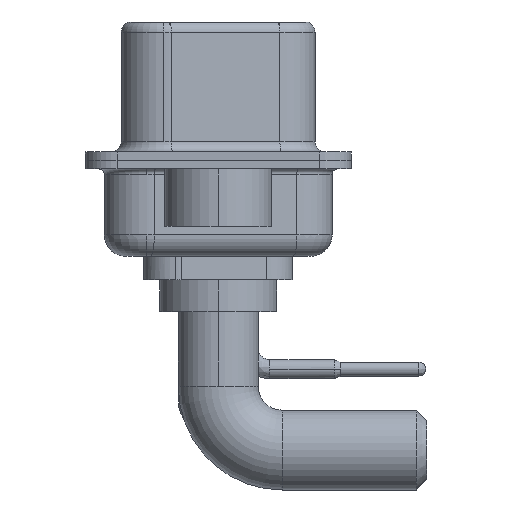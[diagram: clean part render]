
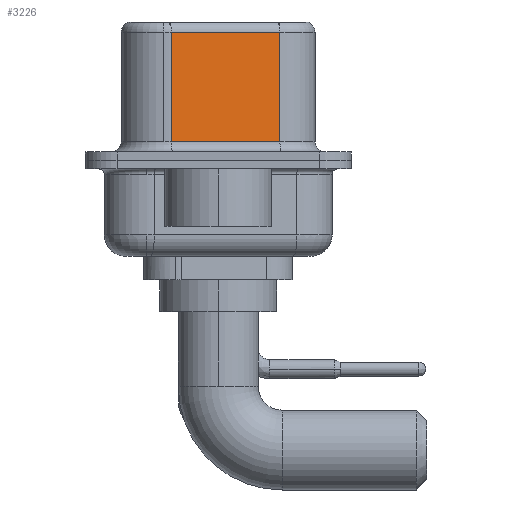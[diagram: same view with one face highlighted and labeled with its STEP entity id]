
A CAD part, left-side view. The second image highlights one B-rep face of the part: STEP entity #3226.
In plain terms, the highlighted planar face has unit normal (-0.985, -0.174, 0).
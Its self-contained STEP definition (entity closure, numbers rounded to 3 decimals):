
#95 = CARTESIAN_POINT ( 'NONE',  ( 4.58, -2.897, 0.9 ) ) ;
#141 = DIRECTION ( 'NONE',  ( 0.985, 0.174, 0. ) ) ;
#1295 = VECTOR ( 'NONE', #1507, 1000. ) ;
#1507 = DIRECTION ( 'NONE',  ( 0., 0., -1. ) ) ;
#2976 = VECTOR ( 'NONE', #14151, 1000. ) ;
#3121 = CARTESIAN_POINT ( 'NONE',  ( 4.58, -2.897, 0.9 ) ) ;
#3226 = ADVANCED_FACE ( 'NONE', ( #17251 ), #7954, .F. ) ;
#4394 = ORIENTED_EDGE ( 'NONE', *, *, #11855, .F. ) ;
#4892 = EDGE_CURVE ( 'NONE', #20461, #14411, #10576, .T. ) ;
#5912 = EDGE_CURVE ( 'NONE', #17487, #20461, #13178, .T. ) ;
#6151 = CARTESIAN_POINT ( 'NONE',  ( 4.58, -2.897, 6.02 ) ) ;
#7954 = PLANE ( 'NONE',  #9165 ) ;
#8474 = LINE ( 'NONE', #3121, #2976 ) ;
#9165 = AXIS2_PLACEMENT_3D ( 'NONE', #10063, #141, #23328 ) ;
#9726 = CARTESIAN_POINT ( 'NONE',  ( 3.68, 2.203, 0.9 ) ) ;
#10063 = CARTESIAN_POINT ( 'NONE',  ( 4.58, -2.897, 6.52 ) ) ;
#10576 = LINE ( 'NONE', #18384, #1295 ) ;
#11517 = CARTESIAN_POINT ( 'NONE',  ( 3.68, 2.203, 6.02 ) ) ;
#11855 = EDGE_CURVE ( 'NONE', #17487, #20853, #12736, .T. ) ;
#12736 = LINE ( 'NONE', #20327, #17567 ) ;
#12982 = DIRECTION ( 'NONE',  ( 0., 0., -1. ) ) ;
#13178 = LINE ( 'NONE', #6151, #18005 ) ;
#14151 = DIRECTION ( 'NONE',  ( 0.174, -0.985, 0. ) ) ;
#14411 = VERTEX_POINT ( 'NONE', #9726 ) ;
#15097 = ORIENTED_EDGE ( 'NONE', *, *, #4892, .T. ) ;
#15219 = EDGE_CURVE ( 'NONE', #14411, #20853, #8474, .T. ) ;
#15337 = ORIENTED_EDGE ( 'NONE', *, *, #5912, .T. ) ;
#17251 = FACE_OUTER_BOUND ( 'NONE', #22195, .T. ) ;
#17487 = VERTEX_POINT ( 'NONE', #18655 ) ;
#17567 = VECTOR ( 'NONE', #12982, 1000. ) ;
#18005 = VECTOR ( 'NONE', #20785, 1000. ) ;
#18384 = CARTESIAN_POINT ( 'NONE',  ( 3.68, 2.203, 6.52 ) ) ;
#18655 = CARTESIAN_POINT ( 'NONE',  ( 4.58, -2.897, 6.02 ) ) ;
#20327 = CARTESIAN_POINT ( 'NONE',  ( 4.58, -2.897, 6.52 ) ) ;
#20384 = ORIENTED_EDGE ( 'NONE', *, *, #15219, .T. ) ;
#20461 = VERTEX_POINT ( 'NONE', #11517 ) ;
#20785 = DIRECTION ( 'NONE',  ( -0.174, 0.985, 0. ) ) ;
#20853 = VERTEX_POINT ( 'NONE', #95 ) ;
#22195 = EDGE_LOOP ( 'NONE', ( #4394, #15337, #15097, #20384 ) ) ;
#23328 = DIRECTION ( 'NONE',  ( -0.174, 0.985, 0. ) ) ;
